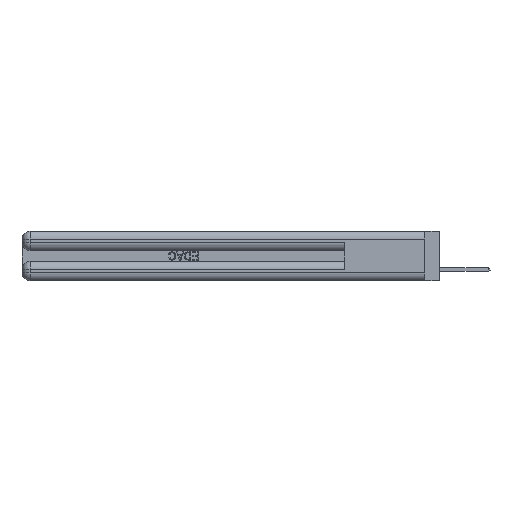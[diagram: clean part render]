
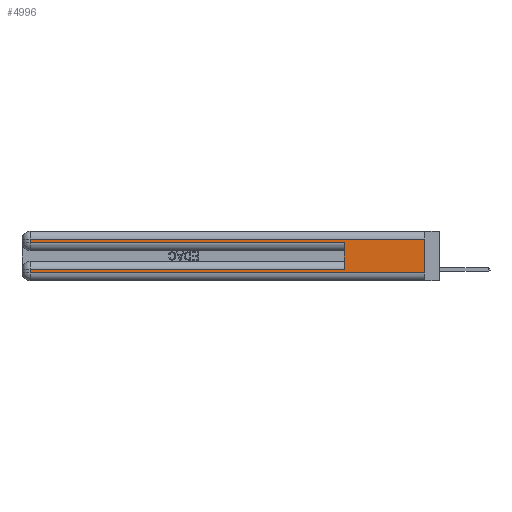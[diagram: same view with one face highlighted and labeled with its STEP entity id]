
A CAD part, left-side view. The second image highlights one B-rep face of the part: STEP entity #4996.
In plain terms, the highlighted planar face has unit normal (-1, 0, 0).
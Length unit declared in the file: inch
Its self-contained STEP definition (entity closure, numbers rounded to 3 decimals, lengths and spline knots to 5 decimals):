
#1184 = VECTOR ( 'NONE', #22240, 39.37008 ) ;
#2065 = DIRECTION ( 'NONE',  ( 0., 1., 0. ) ) ;
#3045 = VERTEX_POINT ( 'NONE', #18228 ) ;
#3597 = ORIENTED_EDGE ( 'NONE', *, *, #30134, .F. ) ;
#4247 = ORIENTED_EDGE ( 'NONE', *, *, #41219, .T. ) ;
#4996 = ADVANCED_FACE ( 'NONE', ( #11789 ), #21581, .F. ) ;
#5129 = LINE ( 'NONE', #39531, #29034 ) ;
#5142 = DIRECTION ( 'NONE',  ( 0., 0., -1. ) ) ;
#6944 = VERTEX_POINT ( 'NONE', #38614 ) ;
#8427 = EDGE_CURVE ( 'NONE', #11782, #10508, #30784, .T. ) ;
#8951 = VERTEX_POINT ( 'NONE', #38080 ) ;
#10073 = DIRECTION ( 'NONE',  ( 0., -1., 0. ) ) ;
#10223 = CARTESIAN_POINT ( 'NONE',  ( 0., 0., 0.285 ) ) ;
#10508 = VERTEX_POINT ( 'NONE', #19798 ) ;
#11245 = EDGE_CURVE ( 'NONE', #6944, #31139, #27924, .T. ) ;
#11258 = CARTESIAN_POINT ( 'NONE',  ( 0., 0., 0.37 ) ) ;
#11308 = VECTOR ( 'NONE', #33579, 39.37008 ) ;
#11692 = DIRECTION ( 'NONE',  ( 1., 0., 0. ) ) ;
#11782 = VERTEX_POINT ( 'NONE', #29106 ) ;
#11789 = FACE_OUTER_BOUND ( 'NONE', #22225, .T. ) ;
#11858 = CARTESIAN_POINT ( 'NONE',  ( 0., 0.6, 0.085 ) ) ;
#12129 = EDGE_CURVE ( 'NONE', #10508, #6944, #31649, .T. ) ;
#12559 = CARTESIAN_POINT ( 'NONE',  ( 0., 0., 0.06 ) ) ;
#12821 = DIRECTION ( 'NONE',  ( 0., 0., -1. ) ) ;
#12874 = CARTESIAN_POINT ( 'NONE',  ( 0., 0.6, 0.285 ) ) ;
#15021 = VERTEX_POINT ( 'NONE', #12559 ) ;
#17180 = VECTOR ( 'NONE', #2065, 39.37008 ) ;
#18228 = CARTESIAN_POINT ( 'NONE',  ( 0., 2.94, 0.085 ) ) ;
#18735 = VERTEX_POINT ( 'NONE', #11858 ) ;
#18944 = LINE ( 'NONE', #39548, #1184 ) ;
#19410 = VECTOR ( 'NONE', #28907, 39.37008 ) ;
#19439 = CARTESIAN_POINT ( 'NONE',  ( 0., 0., 0.31 ) ) ;
#19798 = CARTESIAN_POINT ( 'NONE',  ( 0., 2.94, 0.31 ) ) ;
#21581 = PLANE ( 'NONE',  #36917 ) ;
#22066 = CARTESIAN_POINT ( 'NONE',  ( 0., 0., 0.085 ) ) ;
#22105 = VECTOR ( 'NONE', #10073, 39.37008 ) ;
#22225 = EDGE_LOOP ( 'NONE', ( #34806, #31963, #36428, #29344, #3597, #23555, #24246, #4247 ) ) ;
#22240 = DIRECTION ( 'NONE',  ( 0., 0., -1. ) ) ;
#23510 = DIRECTION ( 'NONE',  ( 0., 0., 1. ) ) ;
#23555 = ORIENTED_EDGE ( 'NONE', *, *, #34349, .T. ) ;
#24246 = ORIENTED_EDGE ( 'NONE', *, *, #35609, .T. ) ;
#24839 = CARTESIAN_POINT ( 'NONE',  ( 0., 2.94, 0.37 ) ) ;
#24973 = EDGE_CURVE ( 'NONE', #11782, #15021, #18944, .T. ) ;
#26456 = CARTESIAN_POINT ( 'NONE',  ( 0., 0.6, 0.145 ) ) ;
#26587 = LINE ( 'NONE', #22066, #17180 ) ;
#27924 = LINE ( 'NONE', #10223, #11308 ) ;
#28907 = DIRECTION ( 'NONE',  ( 0., 1., 0. ) ) ;
#29034 = VECTOR ( 'NONE', #12821, 39.37008 ) ;
#29106 = CARTESIAN_POINT ( 'NONE',  ( 0., 0., 0.31 ) ) ;
#29344 = ORIENTED_EDGE ( 'NONE', *, *, #11245, .T. ) ;
#30134 = EDGE_CURVE ( 'NONE', #18735, #31139, #40856, .T. ) ;
#30784 = LINE ( 'NONE', #19439, #19410 ) ;
#30891 = LINE ( 'NONE', #33293, #22105 ) ;
#31139 = VERTEX_POINT ( 'NONE', #12874 ) ;
#31649 = LINE ( 'NONE', #24839, #37342 ) ;
#31963 = ORIENTED_EDGE ( 'NONE', *, *, #8427, .T. ) ;
#33293 = CARTESIAN_POINT ( 'NONE',  ( 0., 0., 0.06 ) ) ;
#33579 = DIRECTION ( 'NONE',  ( 0., -1., 0. ) ) ;
#34349 = EDGE_CURVE ( 'NONE', #18735, #3045, #26587, .T. ) ;
#34806 = ORIENTED_EDGE ( 'NONE', *, *, #24973, .F. ) ;
#34828 = DIRECTION ( 'NONE',  ( 0., 0., -1. ) ) ;
#35609 = EDGE_CURVE ( 'NONE', #3045, #8951, #5129, .T. ) ;
#35668 = VECTOR ( 'NONE', #23510, 39.37008 ) ;
#36428 = ORIENTED_EDGE ( 'NONE', *, *, #12129, .T. ) ;
#36917 = AXIS2_PLACEMENT_3D ( 'NONE', #11258, #11692, #5142 ) ;
#37342 = VECTOR ( 'NONE', #34828, 39.37008 ) ;
#38080 = CARTESIAN_POINT ( 'NONE',  ( 0., 2.94, 0.06 ) ) ;
#38614 = CARTESIAN_POINT ( 'NONE',  ( 0., 2.94, 0.285 ) ) ;
#39531 = CARTESIAN_POINT ( 'NONE',  ( 0., 2.94, 0.37 ) ) ;
#39548 = CARTESIAN_POINT ( 'NONE',  ( 0., 0., 0.37 ) ) ;
#40856 = LINE ( 'NONE', #26456, #35668 ) ;
#41219 = EDGE_CURVE ( 'NONE', #8951, #15021, #30891, .T. ) ;
